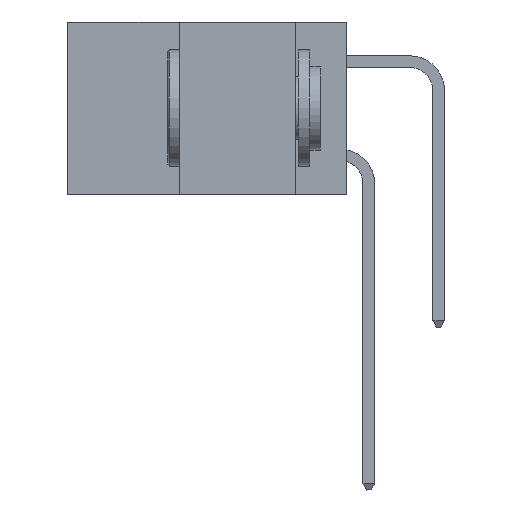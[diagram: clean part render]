
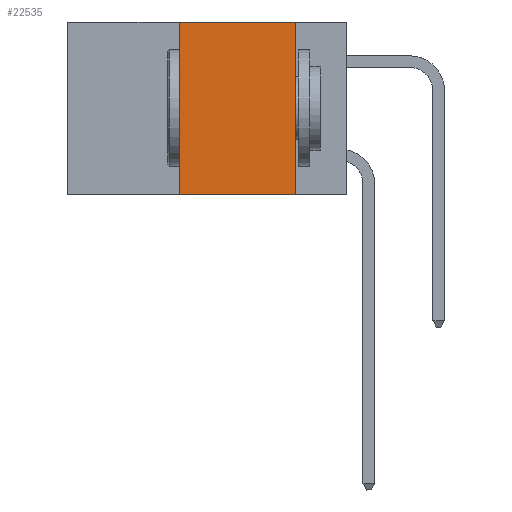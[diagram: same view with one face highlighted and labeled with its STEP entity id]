
A CAD part, left-side view. The second image highlights one B-rep face of the part: STEP entity #22535.
In plain terms, the highlighted planar face has unit normal (-1, 0, 0).
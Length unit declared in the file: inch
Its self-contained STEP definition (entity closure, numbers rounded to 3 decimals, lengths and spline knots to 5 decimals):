
#55 = CARTESIAN_POINT ( 'NONE',  ( 0., 0.11, 0. ) ) ;
#892 = DIRECTION ( 'NONE',  ( 0., -1., 0. ) ) ;
#1624 = DIRECTION ( 'NONE',  ( 0., 0., 1. ) ) ;
#1813 = EDGE_LOOP ( 'NONE', ( #28312, #19112, #20979, #27145 ) ) ;
#2037 = VECTOR ( 'NONE', #892, 39.37008 ) ;
#2043 = EDGE_CURVE ( 'NONE', #14401, #3356, #24394, .T. ) ;
#2095 = LINE ( 'NONE', #20289, #12576 ) ;
#3356 = VERTEX_POINT ( 'NONE', #4467 ) ;
#3409 = VERTEX_POINT ( 'NONE', #55 ) ;
#4467 = CARTESIAN_POINT ( 'NONE',  ( 0., 0.11, -0.37 ) ) ;
#7163 = FACE_OUTER_BOUND ( 'NONE', #1813, .T. ) ;
#8560 = CARTESIAN_POINT ( 'NONE',  ( 0., 0.11, 0. ) ) ;
#8622 = CARTESIAN_POINT ( 'NONE',  ( 0., 0.36, 0. ) ) ;
#11224 = CARTESIAN_POINT ( 'NONE',  ( 0., 0.6, 0. ) ) ;
#12576 = VECTOR ( 'NONE', #1624, 39.37008 ) ;
#12843 = CARTESIAN_POINT ( 'NONE',  ( 0., 0.6, -0.37 ) ) ;
#13553 = LINE ( 'NONE', #21161, #19097 ) ;
#14401 = VERTEX_POINT ( 'NONE', #19147 ) ;
#15186 = VERTEX_POINT ( 'NONE', #8622 ) ;
#15615 = EDGE_CURVE ( 'NONE', #14401, #15186, #2095, .T. ) ;
#18054 = EDGE_CURVE ( 'NONE', #15186, #3409, #13553, .T. ) ;
#18145 = LINE ( 'NONE', #8560, #24564 ) ;
#19097 = VECTOR ( 'NONE', #30843, 39.37008 ) ;
#19112 = ORIENTED_EDGE ( 'NONE', *, *, #18054, .F. ) ;
#19147 = CARTESIAN_POINT ( 'NONE',  ( 0., 0.36, -0.37 ) ) ;
#20289 = CARTESIAN_POINT ( 'NONE',  ( 0., 0.36, 0. ) ) ;
#20733 = DIRECTION ( 'NONE',  ( 0., 0., -1. ) ) ;
#20935 = PLANE ( 'NONE',  #21577 ) ;
#20979 = ORIENTED_EDGE ( 'NONE', *, *, #15615, .F. ) ;
#21161 = CARTESIAN_POINT ( 'NONE',  ( 0., 0.6, 0. ) ) ;
#21577 = AXIS2_PLACEMENT_3D ( 'NONE', #11224, #27724, #20733 ) ;
#22535 = ADVANCED_FACE ( 'NONE', ( #7163 ), #20935, .F. ) ;
#23540 = EDGE_CURVE ( 'NONE', #3409, #3356, #18145, .T. ) ;
#24394 = LINE ( 'NONE', #12843, #2037 ) ;
#24564 = VECTOR ( 'NONE', #27661, 39.37008 ) ;
#27145 = ORIENTED_EDGE ( 'NONE', *, *, #2043, .T. ) ;
#27661 = DIRECTION ( 'NONE',  ( 0., 0., -1. ) ) ;
#27724 = DIRECTION ( 'NONE',  ( 1., 0., 0. ) ) ;
#28312 = ORIENTED_EDGE ( 'NONE', *, *, #23540, .F. ) ;
#30843 = DIRECTION ( 'NONE',  ( 0., -1., 0. ) ) ;
